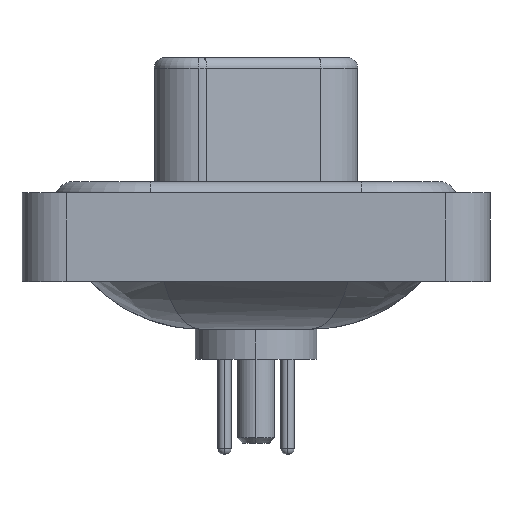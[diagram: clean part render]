
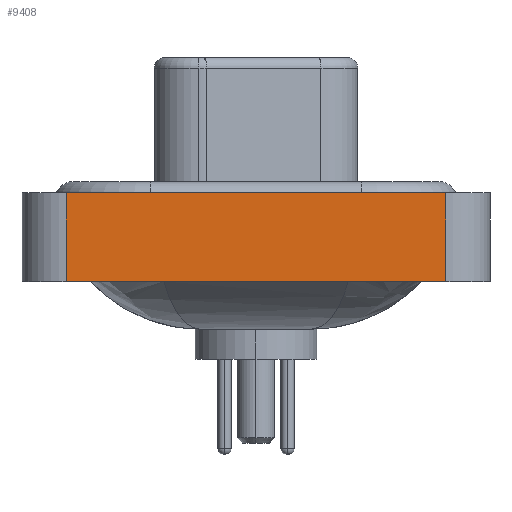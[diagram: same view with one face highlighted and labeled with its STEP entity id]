
A CAD part, left-side view. The second image highlights one B-rep face of the part: STEP entity #9408.
In plain terms, the highlighted planar face has unit normal (-1, 0, 0).
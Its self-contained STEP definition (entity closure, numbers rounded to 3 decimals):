
#261 = VECTOR ( 'NONE', #4060, 1000. ) ;
#1425 = CARTESIAN_POINT ( 'NONE',  ( -7.35, -8.55, -3.6 ) ) ;
#1939 = FACE_OUTER_BOUND ( 'NONE', #4009, .T. ) ;
#3289 = VERTEX_POINT ( 'NONE', #20780 ) ;
#3401 = EDGE_CURVE ( 'NONE', #21453, #14526, #19182, .T. ) ;
#3667 = ORIENTED_EDGE ( 'NONE', *, *, #16958, .T. ) ;
#4009 = EDGE_LOOP ( 'NONE', ( #10531, #10920, #19395, #3667 ) ) ;
#4060 = DIRECTION ( 'NONE',  ( 0., -1., 0. ) ) ;
#4812 = CARTESIAN_POINT ( 'NONE',  ( -7.35, 8.55, -3.6 ) ) ;
#5775 = EDGE_CURVE ( 'NONE', #3289, #15169, #17103, .T. ) ;
#5870 = CARTESIAN_POINT ( 'NONE',  ( -7.35, 8.55, 0.4 ) ) ;
#6180 = DIRECTION ( 'NONE',  ( 0., -1., 0. ) ) ;
#6425 = LINE ( 'NONE', #22336, #14734 ) ;
#7381 = VECTOR ( 'NONE', #15701, 1000. ) ;
#7599 = LINE ( 'NONE', #14809, #261 ) ;
#9130 = PLANE ( 'NONE',  #16399 ) ;
#9408 = ADVANCED_FACE ( 'NONE', ( #1939 ), #9130, .T. ) ;
#10531 = ORIENTED_EDGE ( 'NONE', *, *, #5775, .T. ) ;
#10901 = CARTESIAN_POINT ( 'NONE',  ( -7.35, -8.55, 0.4 ) ) ;
#10920 = ORIENTED_EDGE ( 'NONE', *, *, #13605, .F. ) ;
#11118 = DIRECTION ( 'NONE',  ( 0., 0., 1. ) ) ;
#12781 = CARTESIAN_POINT ( 'NONE',  ( -7.35, -8.55, -3.6 ) ) ;
#13605 = EDGE_CURVE ( 'NONE', #14526, #15169, #7599, .T. ) ;
#14526 = VERTEX_POINT ( 'NONE', #5870 ) ;
#14734 = VECTOR ( 'NONE', #6180, 1000. ) ;
#14809 = CARTESIAN_POINT ( 'NONE',  ( -7.35, -8.55, 0.4 ) ) ;
#15169 = VERTEX_POINT ( 'NONE', #10901 ) ;
#15677 = DIRECTION ( 'NONE',  ( 0., 0., 1. ) ) ;
#15701 = DIRECTION ( 'NONE',  ( 0., 0., 1. ) ) ;
#16399 = AXIS2_PLACEMENT_3D ( 'NONE', #12781, #19950, #11118 ) ;
#16958 = EDGE_CURVE ( 'NONE', #21453, #3289, #6425, .T. ) ;
#17103 = LINE ( 'NONE', #1425, #7381 ) ;
#19182 = LINE ( 'NONE', #4812, #19333 ) ;
#19333 = VECTOR ( 'NONE', #15677, 1000. ) ;
#19395 = ORIENTED_EDGE ( 'NONE', *, *, #3401, .F. ) ;
#19950 = DIRECTION ( 'NONE',  ( -1., 0., 0. ) ) ;
#20049 = CARTESIAN_POINT ( 'NONE',  ( -7.35, 8.55, -3.6 ) ) ;
#20780 = CARTESIAN_POINT ( 'NONE',  ( -7.35, -8.55, -3.6 ) ) ;
#21453 = VERTEX_POINT ( 'NONE', #20049 ) ;
#22336 = CARTESIAN_POINT ( 'NONE',  ( -7.35, -8.55, -3.6 ) ) ;
